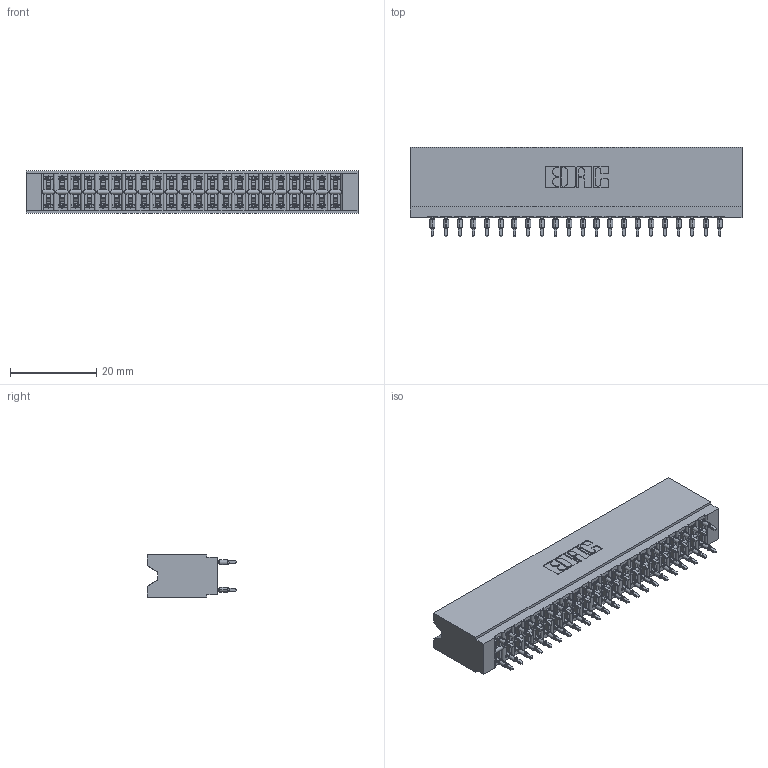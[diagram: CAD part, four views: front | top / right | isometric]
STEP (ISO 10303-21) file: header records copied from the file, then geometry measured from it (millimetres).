
FILE_DESCRIPTION (( 'STEP AP203' ), '1' );
FILE_NAME ('746-044-560-206.STEP', '2026-02-27T15:00:56', ( '' ), ( '' ), 'SwSTEP 2.0', 'SolidWorks 2023', '' );
FILE_SCHEMA (( 'CONFIG_CONTROL_DESIGN' ));
Length unit declared in the file: millimetre
Products named in the file (3): 746-044-560-206; 746 Part_.515 Slot Depth - 06; 746-292-001_560
Assembly tree (45 placements, depth 2):
  746-044-560-206
    746 Part_.515 Slot Depth - 06
    746-292-001_560  x44
Bounding box: 77.09 x 20.82 x 9.91 mm (x, y, z)
Volume: 8521.3 mm3; surface area: 14017.6 mm2
Topology: 45 solids, 45 shells, 4256 faces, 11837 edges, 7589 vertices
Faces by surface type: plane 2124, cylinder 988, bspline 880, torus 264
Entity records: 36980 total; most frequent: CARTESIAN_POINT 7522, ORIENTED_EDGE 6302, DIRECTION 5303, EDGE_CURVE 3151, LINE 2739, VECTOR 2739, VERTEX_POINT 2085, AXIS2_PLACEMENT_3D 1282
